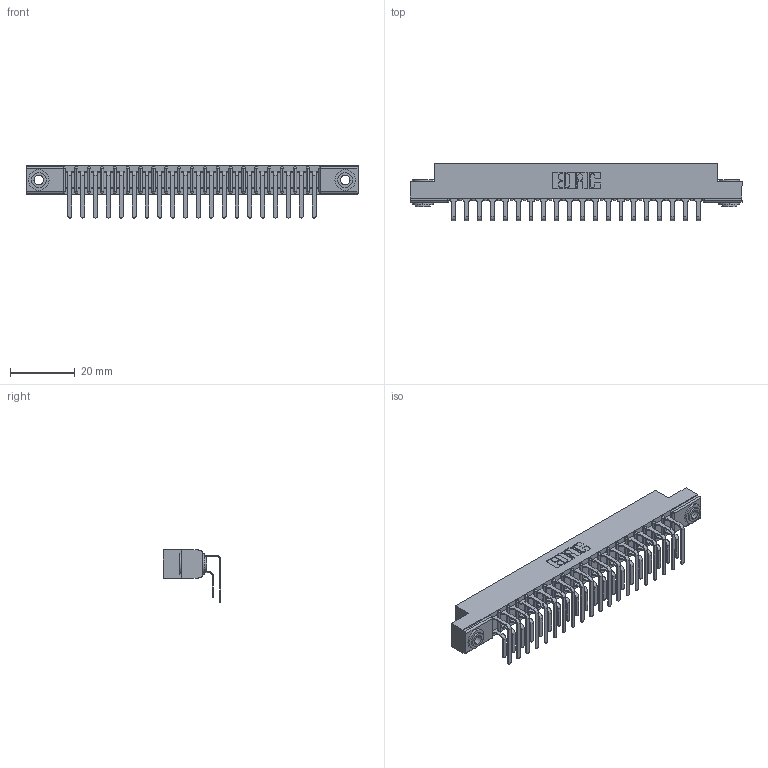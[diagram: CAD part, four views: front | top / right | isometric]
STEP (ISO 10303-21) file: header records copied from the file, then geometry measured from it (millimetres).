
FILE_DESCRIPTION (( 'STEP AP203' ), '1' );
FILE_NAME ('307-020-459-103.STEP', '2020-09-27T02:23:04', ( '' ), ( '' ), 'SwSTEP 2.0', 'SolidWorks 2020', '' );
FILE_SCHEMA (( 'CONFIG_CONTROL_DESIGN' ));
Length unit declared in the file: inch
Products named in the file (5): 307-020-459-103; 307-290-001_559 - 2 (Single); 345-250-002_345-250-002-102; 307 Part_.156 Dia Mounting Holes; 307-290-001_558 559 - 1 (Single)
Assembly tree (43 placements, depth 2):
  307-020-459-103
    307 Part_.156 Dia Mounting Holes
    307-290-001_558 559 - 1 (Single)  x20
    307-290-001_559 - 2 (Single)  x20
    345-250-002_345-250-002-102  x2
Bounding box: 102.26 x 17.69 x 16.08 mm (x, y, z)
Volume: 6867.8 mm3; surface area: 13271.4 mm2
Topology: 43 solids, 43 shells, 2191 faces, 6115 edges, 3962 vertices
Faces by surface type: plane 1414, cylinder 727, sphere 42, cone 8
Entity records: 23010 total; most frequent: CARTESIAN_POINT 3755, ORIENTED_EDGE 3710, DIRECTION 3701, EDGE_CURVE 1855, LINE 1405, VECTOR 1405, VERTEX_POINT 1202, AXIS2_PLACEMENT_3D 1148
